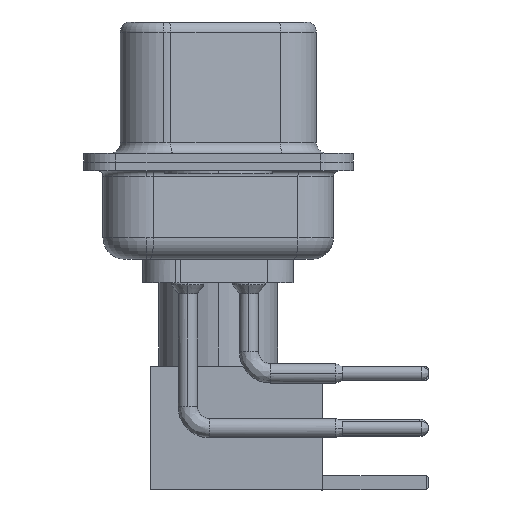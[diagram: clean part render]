
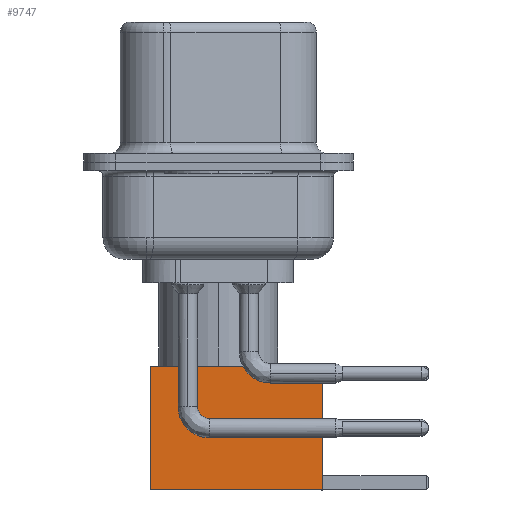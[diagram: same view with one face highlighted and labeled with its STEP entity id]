
A CAD part, left-side view. The second image highlights one B-rep face of the part: STEP entity #9747.
In plain terms, the highlighted face is planar.
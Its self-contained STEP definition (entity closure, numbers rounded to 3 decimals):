
#573 = EDGE_LOOP ( 'NONE', ( #4658, #9387, #21295, #9467 ) ) ;
#2743 = EDGE_CURVE ( 'NONE', #8156, #10441, #20398, .T. ) ;
#2915 = VERTEX_POINT ( 'NONE', #15525 ) ;
#3615 = LINE ( 'NONE', #22471, #22380 ) ;
#4208 = CARTESIAN_POINT ( 'NONE',  ( 2.875, 2.875, 0. ) ) ;
#4460 = EDGE_CURVE ( 'NONE', #5191, #10441, #3615, .T. ) ;
#4658 = ORIENTED_EDGE ( 'NONE', *, *, #6229, .T. ) ;
#5191 = VERTEX_POINT ( 'NONE', #10265 ) ;
#5926 = DIRECTION ( 'NONE',  ( 0., 0., 1. ) ) ;
#5929 = LINE ( 'NONE', #6502, #6307 ) ;
#6229 = EDGE_CURVE ( 'NONE', #2915, #8156, #14397, .T. ) ;
#6307 = VECTOR ( 'NONE', #22806, 1000. ) ;
#6502 = CARTESIAN_POINT ( 'NONE',  ( 0., 2.875, 8. ) ) ;
#7256 = VECTOR ( 'NONE', #21961, 1000. ) ;
#8013 = DIRECTION ( 'NONE',  ( 0., 1., 0. ) ) ;
#8156 = VERTEX_POINT ( 'NONE', #4208 ) ;
#9387 = ORIENTED_EDGE ( 'NONE', *, *, #2743, .T. ) ;
#9467 = ORIENTED_EDGE ( 'NONE', *, *, #16036, .F. ) ;
#9747 = ADVANCED_FACE ( 'NONE', ( #21418 ), #17327, .T. ) ;
#10265 = CARTESIAN_POINT ( 'NONE',  ( -2.875, 2.875, 8. ) ) ;
#10441 = VERTEX_POINT ( 'NONE', #20265 ) ;
#12170 = CARTESIAN_POINT ( 'NONE',  ( 2.875, 2.875, 0. ) ) ;
#14397 = LINE ( 'NONE', #12170, #7256 ) ;
#15061 = CARTESIAN_POINT ( 'NONE',  ( 0., 2.875, 0. ) ) ;
#15525 = CARTESIAN_POINT ( 'NONE',  ( 2.875, 2.875, 8. ) ) ;
#16036 = EDGE_CURVE ( 'NONE', #2915, #5191, #5929, .T. ) ;
#16833 = VECTOR ( 'NONE', #22247, 1000. ) ;
#17327 = PLANE ( 'NONE',  #22034 ) ;
#20245 = DIRECTION ( 'NONE',  ( 0., 0., -1. ) ) ;
#20265 = CARTESIAN_POINT ( 'NONE',  ( -2.875, 2.875, 0. ) ) ;
#20398 = LINE ( 'NONE', #15061, #16833 ) ;
#21295 = ORIENTED_EDGE ( 'NONE', *, *, #4460, .F. ) ;
#21418 = FACE_OUTER_BOUND ( 'NONE', #573, .T. ) ;
#21961 = DIRECTION ( 'NONE',  ( 0., 0., -1. ) ) ;
#22034 = AXIS2_PLACEMENT_3D ( 'NONE', #23044, #8013, #5926 ) ;
#22247 = DIRECTION ( 'NONE',  ( -1., 0., 0. ) ) ;
#22380 = VECTOR ( 'NONE', #20245, 1000. ) ;
#22471 = CARTESIAN_POINT ( 'NONE',  ( -2.875, 2.875, 0. ) ) ;
#22806 = DIRECTION ( 'NONE',  ( -1., 0., 0. ) ) ;
#23044 = CARTESIAN_POINT ( 'NONE',  ( 2.875, 2.875, 0. ) ) ;
